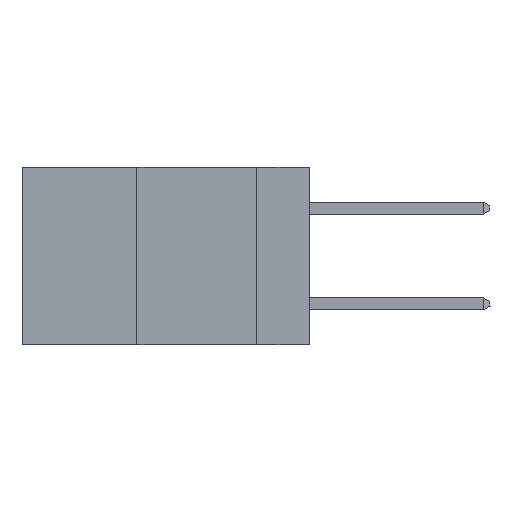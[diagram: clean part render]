
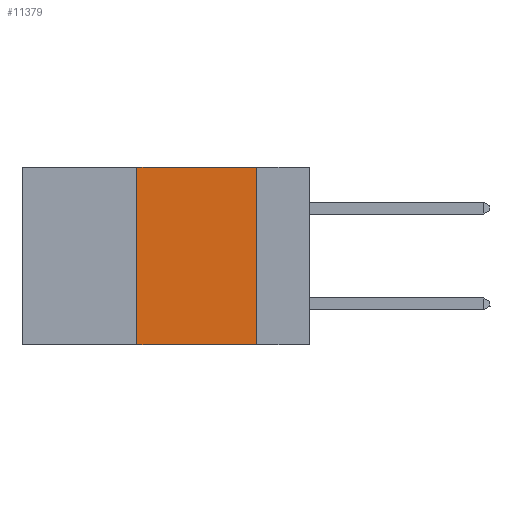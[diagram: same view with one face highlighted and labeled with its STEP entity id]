
A CAD part, left-side view. The second image highlights one B-rep face of the part: STEP entity #11379.
In plain terms, the highlighted planar face has unit normal (-1, 0, 0).
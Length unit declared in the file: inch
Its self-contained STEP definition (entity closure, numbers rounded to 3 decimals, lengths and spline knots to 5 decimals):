
#814 = DIRECTION ( 'NONE',  ( 0., -1., 0. ) ) ;
#1084 = LINE ( 'NONE', #17550, #11390 ) ;
#1252 = CARTESIAN_POINT ( 'NONE',  ( 0., 0.6, -0.37 ) ) ;
#1605 = DIRECTION ( 'NONE',  ( 0., 0., -1. ) ) ;
#1877 = LINE ( 'NONE', #11493, #4770 ) ;
#2290 = CARTESIAN_POINT ( 'NONE',  ( 0., 0.36, 0. ) ) ;
#3065 = ORIENTED_EDGE ( 'NONE', *, *, #14388, .F. ) ;
#3466 = AXIS2_PLACEMENT_3D ( 'NONE', #16869, #9965, #1605 ) ;
#3938 = ORIENTED_EDGE ( 'NONE', *, *, #15282, .T. ) ;
#4741 = VECTOR ( 'NONE', #11033, 39.37008 ) ;
#4770 = VECTOR ( 'NONE', #12903, 39.37008 ) ;
#5433 = VERTEX_POINT ( 'NONE', #7704 ) ;
#5469 = ORIENTED_EDGE ( 'NONE', *, *, #15405, .F. ) ;
#5843 = VECTOR ( 'NONE', #11342, 39.37008 ) ;
#6204 = CARTESIAN_POINT ( 'NONE',  ( 0., 0.11, 0. ) ) ;
#6285 = LINE ( 'NONE', #7220, #5843 ) ;
#7220 = CARTESIAN_POINT ( 'NONE',  ( 0., 0.36, 0. ) ) ;
#7227 = PLANE ( 'NONE',  #3466 ) ;
#7413 = ORIENTED_EDGE ( 'NONE', *, *, #12850, .F. ) ;
#7445 = FACE_OUTER_BOUND ( 'NONE', #11025, .T. ) ;
#7704 = CARTESIAN_POINT ( 'NONE',  ( 0., 0.36, -0.37 ) ) ;
#9297 = VERTEX_POINT ( 'NONE', #6204 ) ;
#9861 = VERTEX_POINT ( 'NONE', #12909 ) ;
#9965 = DIRECTION ( 'NONE',  ( 1., 0., 0. ) ) ;
#11025 = EDGE_LOOP ( 'NONE', ( #7413, #3065, #5469, #3938 ) ) ;
#11033 = DIRECTION ( 'NONE',  ( 0., -1., 0. ) ) ;
#11342 = DIRECTION ( 'NONE',  ( 0., 0., 1. ) ) ;
#11379 = ADVANCED_FACE ( 'NONE', ( #7445 ), #7227, .F. ) ;
#11390 = VECTOR ( 'NONE', #814, 39.37008 ) ;
#11493 = CARTESIAN_POINT ( 'NONE',  ( 0., 0.11, 0. ) ) ;
#11644 = LINE ( 'NONE', #1252, #4741 ) ;
#12850 = EDGE_CURVE ( 'NONE', #9297, #9861, #1877, .T. ) ;
#12903 = DIRECTION ( 'NONE',  ( 0., 0., -1. ) ) ;
#12909 = CARTESIAN_POINT ( 'NONE',  ( 0., 0.11, -0.37 ) ) ;
#13714 = VERTEX_POINT ( 'NONE', #2290 ) ;
#14388 = EDGE_CURVE ( 'NONE', #13714, #9297, #1084, .T. ) ;
#15282 = EDGE_CURVE ( 'NONE', #5433, #9861, #11644, .T. ) ;
#15405 = EDGE_CURVE ( 'NONE', #5433, #13714, #6285, .T. ) ;
#16869 = CARTESIAN_POINT ( 'NONE',  ( 0., 0.6, 0. ) ) ;
#17550 = CARTESIAN_POINT ( 'NONE',  ( 0., 0.6, 0. ) ) ;
